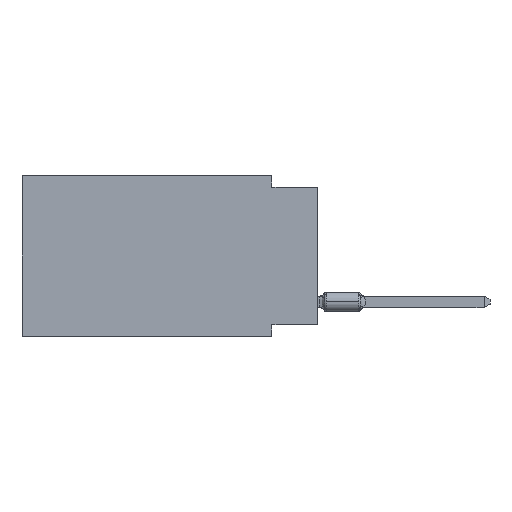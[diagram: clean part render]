
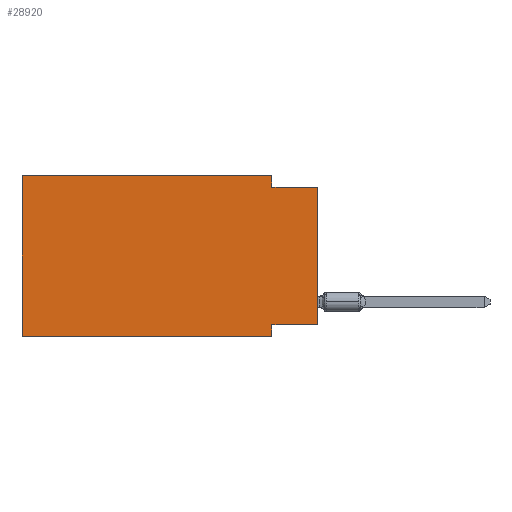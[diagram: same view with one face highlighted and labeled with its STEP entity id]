
A CAD part, left-side view. The second image highlights one B-rep face of the part: STEP entity #28920.
In plain terms, the highlighted planar face has unit normal (-1, 0, 0).
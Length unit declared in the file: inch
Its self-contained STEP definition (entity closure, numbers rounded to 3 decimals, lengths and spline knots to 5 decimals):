
#555 = ORIENTED_EDGE ( 'NONE', *, *, #14324, .F. ) ;
#564 = CARTESIAN_POINT ( 'NONE',  ( 0., 0., -0.025 ) ) ;
#1387 = EDGE_CURVE ( 'NONE', #33727, #20189, #34906, .T. ) ;
#1546 = DIRECTION ( 'NONE',  ( 0., 1., 0. ) ) ;
#2316 = CARTESIAN_POINT ( 'NONE',  ( 0., 0.1, -0.325 ) ) ;
#2940 = CARTESIAN_POINT ( 'NONE',  ( 0., 0.645, -0.35 ) ) ;
#3151 = CARTESIAN_POINT ( 'NONE',  ( 0., 0.645, 0. ) ) ;
#3543 = CARTESIAN_POINT ( 'NONE',  ( 0., 0.1, 0. ) ) ;
#4195 = VECTOR ( 'NONE', #20239, 39.37008 ) ;
#4377 = AXIS2_PLACEMENT_3D ( 'NONE', #15072, #24706, #37461 ) ;
#6264 = CARTESIAN_POINT ( 'NONE',  ( 0., 0.1, 0. ) ) ;
#6326 = CARTESIAN_POINT ( 'NONE',  ( 0., 0.645, -0.35 ) ) ;
#6482 = DIRECTION ( 'NONE',  ( 0., -1., 0. ) ) ;
#6949 = EDGE_CURVE ( 'NONE', #33112, #33727, #13355, .T. ) ;
#7455 = VERTEX_POINT ( 'NONE', #36879 ) ;
#8659 = EDGE_CURVE ( 'NONE', #20189, #22286, #17819, .T. ) ;
#8844 = CARTESIAN_POINT ( 'NONE',  ( 0., 0.1, -0.35 ) ) ;
#9982 = VECTOR ( 'NONE', #25489, 39.37008 ) ;
#10932 = LINE ( 'NONE', #17203, #29689 ) ;
#12101 = VERTEX_POINT ( 'NONE', #2316 ) ;
#12951 = ORIENTED_EDGE ( 'NONE', *, *, #8659, .F. ) ;
#13355 = LINE ( 'NONE', #3151, #25550 ) ;
#14324 = EDGE_CURVE ( 'NONE', #12101, #7455, #31023, .T. ) ;
#15072 = CARTESIAN_POINT ( 'NONE',  ( 0., 0.645, 0. ) ) ;
#15255 = DIRECTION ( 'NONE',  ( 0., -1., 0. ) ) ;
#15332 = EDGE_CURVE ( 'NONE', #17949, #7455, #40782, .T. ) ;
#17203 = CARTESIAN_POINT ( 'NONE',  ( 0., 0., -0.325 ) ) ;
#17622 = EDGE_CURVE ( 'NONE', #33142, #22286, #39369, .T. ) ;
#17819 = LINE ( 'NONE', #564, #28108 ) ;
#17949 = VERTEX_POINT ( 'NONE', #6326 ) ;
#18379 = VECTOR ( 'NONE', #15255, 39.37008 ) ;
#18524 = EDGE_CURVE ( 'NONE', #17949, #33112, #28828, .T. ) ;
#19719 = CARTESIAN_POINT ( 'NONE',  ( 0., 0., 0. ) ) ;
#20189 = VERTEX_POINT ( 'NONE', #38644 ) ;
#20239 = DIRECTION ( 'NONE',  ( 0., 0., 1. ) ) ;
#21931 = ORIENTED_EDGE ( 'NONE', *, *, #17622, .T. ) ;
#22286 = VERTEX_POINT ( 'NONE', #38131 ) ;
#23228 = ORIENTED_EDGE ( 'NONE', *, *, #1387, .F. ) ;
#24530 = DIRECTION ( 'NONE',  ( 0., 0., -1. ) ) ;
#24706 = DIRECTION ( 'NONE',  ( 1., 0., 0. ) ) ;
#25489 = DIRECTION ( 'NONE',  ( 0., 0., -1. ) ) ;
#25550 = VECTOR ( 'NONE', #6482, 39.37008 ) ;
#26511 = ORIENTED_EDGE ( 'NONE', *, *, #18524, .F. ) ;
#26933 = CARTESIAN_POINT ( 'NONE',  ( 0., 0.645, 0. ) ) ;
#27034 = DIRECTION ( 'NONE',  ( 0., -1., 0. ) ) ;
#27911 = EDGE_CURVE ( 'NONE', #33142, #12101, #10932, .T. ) ;
#28108 = VECTOR ( 'NONE', #27034, 39.37008 ) ;
#28291 = CARTESIAN_POINT ( 'NONE',  ( 0., 0.645, 0. ) ) ;
#28828 = LINE ( 'NONE', #26933, #4195 ) ;
#28920 = ADVANCED_FACE ( 'NONE', ( #37865 ), #40166, .F. ) ;
#28956 = VECTOR ( 'NONE', #32697, 39.37008 ) ;
#29689 = VECTOR ( 'NONE', #1546, 39.37008 ) ;
#31023 = LINE ( 'NONE', #8844, #32362 ) ;
#32362 = VECTOR ( 'NONE', #24530, 39.37008 ) ;
#32697 = DIRECTION ( 'NONE',  ( 0., 0., 1. ) ) ;
#32967 = ORIENTED_EDGE ( 'NONE', *, *, #15332, .T. ) ;
#33112 = VERTEX_POINT ( 'NONE', #28291 ) ;
#33142 = VERTEX_POINT ( 'NONE', #37281 ) ;
#33727 = VERTEX_POINT ( 'NONE', #3543 ) ;
#34078 = ORIENTED_EDGE ( 'NONE', *, *, #27911, .F. ) ;
#34906 = LINE ( 'NONE', #6264, #9982 ) ;
#36879 = CARTESIAN_POINT ( 'NONE',  ( 0., 0.1, -0.35 ) ) ;
#37281 = CARTESIAN_POINT ( 'NONE',  ( 0., 0., -0.325 ) ) ;
#37461 = DIRECTION ( 'NONE',  ( 0., 0., -1. ) ) ;
#37865 = FACE_OUTER_BOUND ( 'NONE', #41196, .T. ) ;
#38131 = CARTESIAN_POINT ( 'NONE',  ( 0., 0., -0.025 ) ) ;
#38644 = CARTESIAN_POINT ( 'NONE',  ( 0., 0.1, -0.025 ) ) ;
#39369 = LINE ( 'NONE', #19719, #28956 ) ;
#40166 = PLANE ( 'NONE',  #4377 ) ;
#40726 = ORIENTED_EDGE ( 'NONE', *, *, #6949, .F. ) ;
#40782 = LINE ( 'NONE', #2940, #18379 ) ;
#41196 = EDGE_LOOP ( 'NONE', ( #21931, #12951, #23228, #40726, #26511, #32967, #555, #34078 ) ) ;
